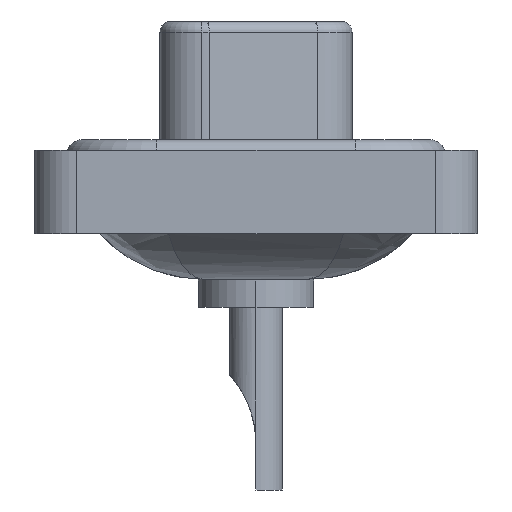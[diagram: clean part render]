
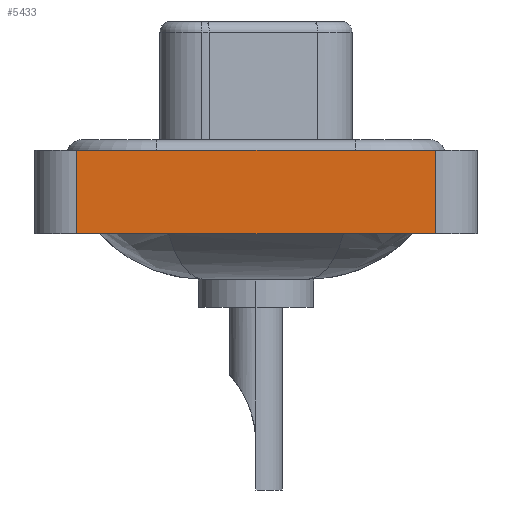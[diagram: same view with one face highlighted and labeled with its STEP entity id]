
A CAD part, left-side view. The second image highlights one B-rep face of the part: STEP entity #5433.
In plain terms, the highlighted planar face has unit normal (-1, 0, 0).
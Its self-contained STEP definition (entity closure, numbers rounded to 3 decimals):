
#956 = DIRECTION ( 'NONE',  ( -1., 0., 0. ) ) ;
#1095 = EDGE_CURVE ( 'NONE', #5258, #1493, #3103, .T. ) ;
#1493 = VERTEX_POINT ( 'NONE', #8753 ) ;
#2061 = DIRECTION ( 'NONE',  ( 0., 0., 1. ) ) ;
#2234 = EDGE_LOOP ( 'NONE', ( #18084, #3633, #3859, #17229 ) ) ;
#3103 = LINE ( 'NONE', #5800, #7747 ) ;
#3633 = ORIENTED_EDGE ( 'NONE', *, *, #14419, .F. ) ;
#3706 = CARTESIAN_POINT ( 'NONE',  ( -7.35, -8.55, -3.6 ) ) ;
#3859 = ORIENTED_EDGE ( 'NONE', *, *, #16490, .F. ) ;
#3980 = LINE ( 'NONE', #7978, #8820 ) ;
#4814 = LINE ( 'NONE', #3706, #6915 ) ;
#4909 = EDGE_CURVE ( 'NONE', #15442, #5258, #4814, .T. ) ;
#5258 = VERTEX_POINT ( 'NONE', #5814 ) ;
#5344 = PLANE ( 'NONE',  #17032 ) ;
#5433 = ADVANCED_FACE ( 'NONE', ( #12479 ), #5344, .T. ) ;
#5679 = CARTESIAN_POINT ( 'NONE',  ( -7.35, 8.55, -3.6 ) ) ;
#5800 = CARTESIAN_POINT ( 'NONE',  ( -7.35, -8.55, -3.6 ) ) ;
#5814 = CARTESIAN_POINT ( 'NONE',  ( -7.35, -8.55, -3.6 ) ) ;
#6247 = CARTESIAN_POINT ( 'NONE',  ( -7.35, 8.55, -3.6 ) ) ;
#6574 = DIRECTION ( 'NONE',  ( 0., -1., 0. ) ) ;
#6915 = VECTOR ( 'NONE', #7786, 1000. ) ;
#7747 = VECTOR ( 'NONE', #11645, 1000. ) ;
#7786 = DIRECTION ( 'NONE',  ( 0., -1., 0. ) ) ;
#7978 = CARTESIAN_POINT ( 'NONE',  ( -7.35, -8.55, 0.4 ) ) ;
#8753 = CARTESIAN_POINT ( 'NONE',  ( -7.35, -8.55, 0.4 ) ) ;
#8820 = VECTOR ( 'NONE', #6574, 1000. ) ;
#9436 = CARTESIAN_POINT ( 'NONE',  ( -7.35, -8.55, -3.6 ) ) ;
#11645 = DIRECTION ( 'NONE',  ( 0., 0., 1. ) ) ;
#11827 = LINE ( 'NONE', #6247, #11841 ) ;
#11841 = VECTOR ( 'NONE', #2061, 1000. ) ;
#12479 = FACE_OUTER_BOUND ( 'NONE', #2234, .T. ) ;
#13787 = DIRECTION ( 'NONE',  ( 0., 0., 1. ) ) ;
#14419 = EDGE_CURVE ( 'NONE', #17538, #1493, #3980, .T. ) ;
#15442 = VERTEX_POINT ( 'NONE', #5679 ) ;
#16490 = EDGE_CURVE ( 'NONE', #15442, #17538, #11827, .T. ) ;
#17032 = AXIS2_PLACEMENT_3D ( 'NONE', #9436, #956, #13787 ) ;
#17229 = ORIENTED_EDGE ( 'NONE', *, *, #4909, .T. ) ;
#17538 = VERTEX_POINT ( 'NONE', #17563 ) ;
#17563 = CARTESIAN_POINT ( 'NONE',  ( -7.35, 8.55, 0.4 ) ) ;
#18084 = ORIENTED_EDGE ( 'NONE', *, *, #1095, .T. ) ;
